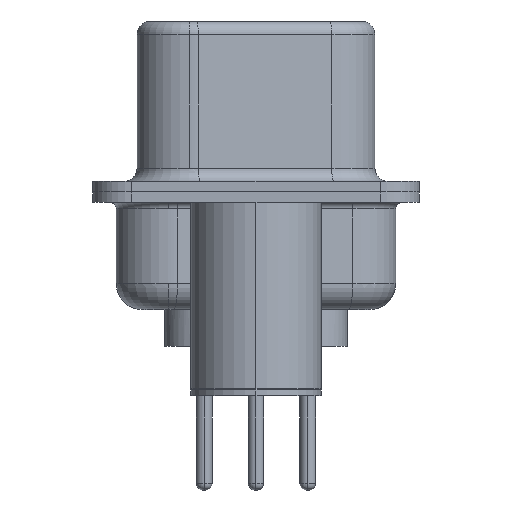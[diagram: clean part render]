
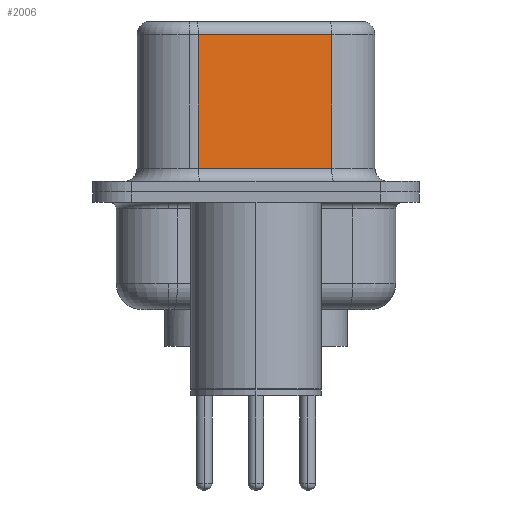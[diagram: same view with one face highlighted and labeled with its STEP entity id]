
A CAD part, left-side view. The second image highlights one B-rep face of the part: STEP entity #2006.
In plain terms, the highlighted planar face has unit normal (-0.985, -0.174, 0).
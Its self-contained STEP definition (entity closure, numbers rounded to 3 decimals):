
#49 = VECTOR ( 'NONE', #14112, 1000. ) ;
#206 = VECTOR ( 'NONE', #592, 1000. ) ;
#266 = CARTESIAN_POINT ( 'NONE',  ( 4.555, -2.897, 6.02 ) ) ;
#592 = DIRECTION ( 'NONE',  ( 0., 0., -1. ) ) ;
#2006 = ADVANCED_FACE ( 'NONE', ( #9574 ), #3966, .F. ) ;
#2446 = DIRECTION ( 'NONE',  ( -0.174, 0.985, 0. ) ) ;
#3934 = DIRECTION ( 'NONE',  ( 0.985, 0.174, 0. ) ) ;
#3966 = PLANE ( 'NONE',  #5508 ) ;
#4192 = CARTESIAN_POINT ( 'NONE',  ( 4.555, -2.897, 6.52 ) ) ;
#4753 = LINE ( 'NONE', #10670, #206 ) ;
#5508 = AXIS2_PLACEMENT_3D ( 'NONE', #4192, #3934, #2446 ) ;
#5845 = CARTESIAN_POINT ( 'NONE',  ( 4.555, -2.897, 0.9 ) ) ;
#6457 = EDGE_LOOP ( 'NONE', ( #11110, #20533, #8446, #12703 ) ) ;
#8109 = CARTESIAN_POINT ( 'NONE',  ( 3.655, 2.203, 6.02 ) ) ;
#8446 = ORIENTED_EDGE ( 'NONE', *, *, #17292, .T. ) ;
#9574 = FACE_OUTER_BOUND ( 'NONE', #6457, .T. ) ;
#10670 = CARTESIAN_POINT ( 'NONE',  ( 4.555, -2.897, 6.52 ) ) ;
#11110 = ORIENTED_EDGE ( 'NONE', *, *, #18199, .F. ) ;
#11223 = DIRECTION ( 'NONE',  ( 0., 0., -1. ) ) ;
#12025 = DIRECTION ( 'NONE',  ( -0.174, 0.985, 0. ) ) ;
#12085 = VERTEX_POINT ( 'NONE', #18814 ) ;
#12703 = ORIENTED_EDGE ( 'NONE', *, *, #13160, .T. ) ;
#13160 = EDGE_CURVE ( 'NONE', #18726, #13570, #14452, .T. ) ;
#13570 = VERTEX_POINT ( 'NONE', #13594 ) ;
#13594 = CARTESIAN_POINT ( 'NONE',  ( 4.555, -2.897, 0.9 ) ) ;
#14112 = DIRECTION ( 'NONE',  ( 0.174, -0.985, 0. ) ) ;
#14452 = LINE ( 'NONE', #5845, #49 ) ;
#14588 = LINE ( 'NONE', #19236, #18313 ) ;
#15126 = EDGE_CURVE ( 'NONE', #12085, #19925, #19391, .T. ) ;
#16879 = CARTESIAN_POINT ( 'NONE',  ( 3.655, 2.203, 0.9 ) ) ;
#17292 = EDGE_CURVE ( 'NONE', #19925, #18726, #14588, .T. ) ;
#18199 = EDGE_CURVE ( 'NONE', #12085, #13570, #4753, .T. ) ;
#18313 = VECTOR ( 'NONE', #11223, 1000. ) ;
#18726 = VERTEX_POINT ( 'NONE', #16879 ) ;
#18814 = CARTESIAN_POINT ( 'NONE',  ( 4.555, -2.897, 6.02 ) ) ;
#19236 = CARTESIAN_POINT ( 'NONE',  ( 3.655, 2.203, 6.52 ) ) ;
#19391 = LINE ( 'NONE', #266, #19892 ) ;
#19892 = VECTOR ( 'NONE', #12025, 1000. ) ;
#19925 = VERTEX_POINT ( 'NONE', #8109 ) ;
#20533 = ORIENTED_EDGE ( 'NONE', *, *, #15126, .T. ) ;
